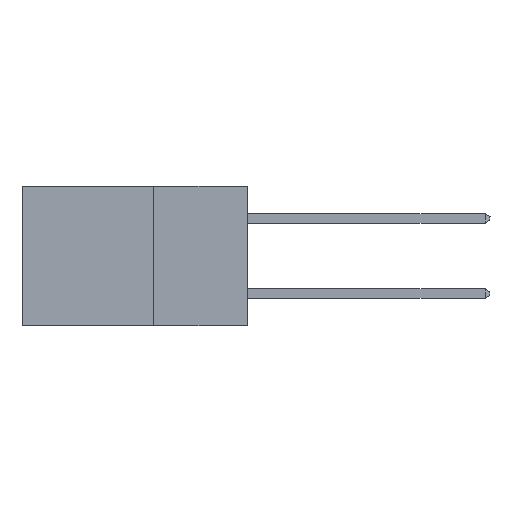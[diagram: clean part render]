
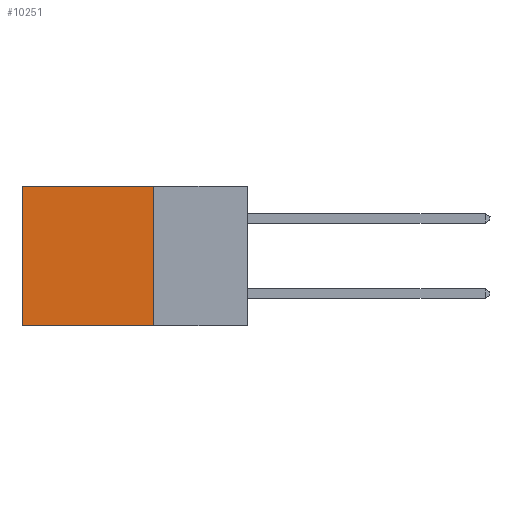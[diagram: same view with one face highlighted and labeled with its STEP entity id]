
A CAD part, left-side view. The second image highlights one B-rep face of the part: STEP entity #10251.
In plain terms, the highlighted planar face has unit normal (-1, 0, 0).
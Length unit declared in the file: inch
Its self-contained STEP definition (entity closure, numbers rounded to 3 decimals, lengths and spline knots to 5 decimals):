
#1 = LINE ( 'NONE', #3509, #7107 ) ;
#381 = EDGE_CURVE ( 'NONE', #9151, #2535, #1, .T. ) ;
#1018 = ORIENTED_EDGE ( 'NONE', *, *, #7228, .F. ) ;
#1125 = DIRECTION ( 'NONE',  ( 0., 0., -1. ) ) ;
#1277 = VECTOR ( 'NONE', #1645, 39.37008 ) ;
#1580 = CARTESIAN_POINT ( 'NONE',  ( 0.2615, 0.25, -0.37 ) ) ;
#1645 = DIRECTION ( 'NONE',  ( 0., 0., -1. ) ) ;
#1816 = DIRECTION ( 'NONE',  ( 0., 1., 0. ) ) ;
#2377 = CARTESIAN_POINT ( 'NONE',  ( 0.2615, 0.6, 0. ) ) ;
#2535 = VERTEX_POINT ( 'NONE', #13162 ) ;
#3182 = VERTEX_POINT ( 'NONE', #8136 ) ;
#3287 = PLANE ( 'NONE',  #10764 ) ;
#3509 = CARTESIAN_POINT ( 'NONE',  ( 0.2615, 0.6, -0.37 ) ) ;
#3933 = ORIENTED_EDGE ( 'NONE', *, *, #12545, .T. ) ;
#3971 = FACE_OUTER_BOUND ( 'NONE', #9149, .T. ) ;
#4394 = DIRECTION ( 'NONE',  ( 0., 1., 0. ) ) ;
#5232 = LINE ( 'NONE', #9756, #9949 ) ;
#5379 = DIRECTION ( 'NONE',  ( 1., 0., 0. ) ) ;
#5495 = CARTESIAN_POINT ( 'NONE',  ( 0.2615, 0.25, 0. ) ) ;
#7107 = VECTOR ( 'NONE', #1125, 39.37008 ) ;
#7228 = EDGE_CURVE ( 'NONE', #3182, #10142, #10664, .T. ) ;
#7718 = LINE ( 'NONE', #5495, #11286 ) ;
#7826 = CARTESIAN_POINT ( 'NONE',  ( 0.2615, 0.25, -0.37 ) ) ;
#8136 = CARTESIAN_POINT ( 'NONE',  ( 0.2615, 0.25, 0. ) ) ;
#8927 = EDGE_CURVE ( 'NONE', #10142, #2535, #5232, .T. ) ;
#9149 = EDGE_LOOP ( 'NONE', ( #13726, #11224, #1018, #3933 ) ) ;
#9151 = VERTEX_POINT ( 'NONE', #2377 ) ;
#9756 = CARTESIAN_POINT ( 'NONE',  ( 0.2615, 0.25, -0.37 ) ) ;
#9949 = VECTOR ( 'NONE', #4394, 39.37008 ) ;
#10142 = VERTEX_POINT ( 'NONE', #1580 ) ;
#10251 = ADVANCED_FACE ( 'NONE', ( #3971 ), #3287, .F. ) ;
#10664 = LINE ( 'NONE', #14172, #1277 ) ;
#10764 = AXIS2_PLACEMENT_3D ( 'NONE', #7826, #5379, #13339 ) ;
#11224 = ORIENTED_EDGE ( 'NONE', *, *, #8927, .F. ) ;
#11286 = VECTOR ( 'NONE', #1816, 39.37008 ) ;
#12545 = EDGE_CURVE ( 'NONE', #3182, #9151, #7718, .T. ) ;
#13162 = CARTESIAN_POINT ( 'NONE',  ( 0.2615, 0.6, -0.37 ) ) ;
#13339 = DIRECTION ( 'NONE',  ( 0., 0., -1. ) ) ;
#13726 = ORIENTED_EDGE ( 'NONE', *, *, #381, .T. ) ;
#14172 = CARTESIAN_POINT ( 'NONE',  ( 0.2615, 0.25, -0.37 ) ) ;
